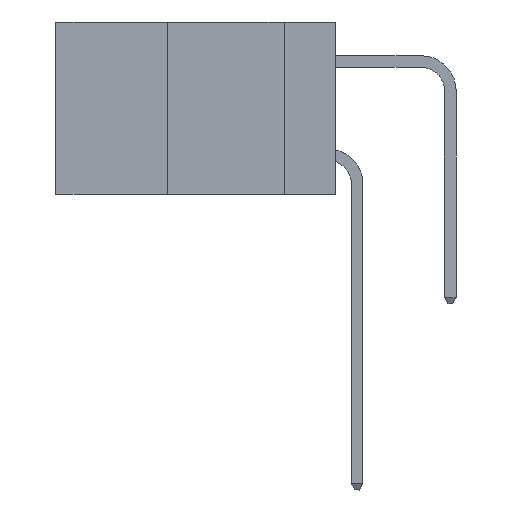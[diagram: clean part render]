
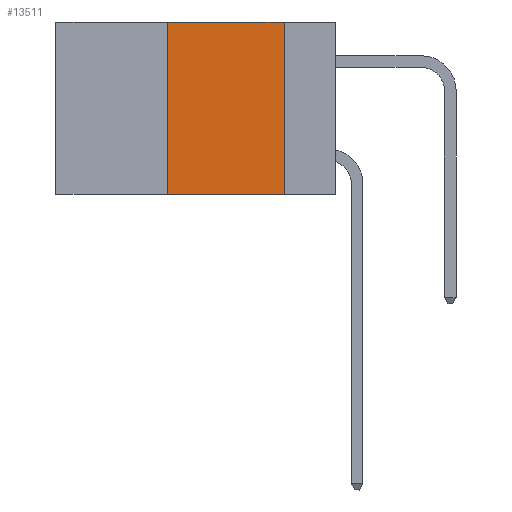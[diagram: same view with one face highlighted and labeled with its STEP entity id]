
A CAD part, left-side view. The second image highlights one B-rep face of the part: STEP entity #13511.
In plain terms, the highlighted planar face has unit normal (-1, 0, 0).
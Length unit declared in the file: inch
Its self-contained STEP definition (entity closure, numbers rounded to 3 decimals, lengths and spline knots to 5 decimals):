
#1411 = EDGE_CURVE ( 'NONE', #8501, #7712, #13005, .T. ) ;
#2580 = CARTESIAN_POINT ( 'NONE',  ( 0., 0.11, 0. ) ) ;
#2696 = LINE ( 'NONE', #4878, #17691 ) ;
#2960 = CARTESIAN_POINT ( 'NONE',  ( 0., 0.6, -0.37 ) ) ;
#3061 = DIRECTION ( 'NONE',  ( 1., 0., 0. ) ) ;
#4762 = AXIS2_PLACEMENT_3D ( 'NONE', #6538, #3061, #13594 ) ;
#4878 = CARTESIAN_POINT ( 'NONE',  ( 0., 0.6, 0. ) ) ;
#6538 = CARTESIAN_POINT ( 'NONE',  ( 0., 0.6, 0. ) ) ;
#7712 = VERTEX_POINT ( 'NONE', #12210 ) ;
#8501 = VERTEX_POINT ( 'NONE', #11268 ) ;
#8573 = DIRECTION ( 'NONE',  ( 0., 0., -1. ) ) ;
#8809 = VERTEX_POINT ( 'NONE', #17375 ) ;
#9532 = EDGE_CURVE ( 'NONE', #8501, #8809, #18796, .T. ) ;
#11268 = CARTESIAN_POINT ( 'NONE',  ( 0., 0.36, -0.37 ) ) ;
#12210 = CARTESIAN_POINT ( 'NONE',  ( 0., 0.36, 0. ) ) ;
#13005 = LINE ( 'NONE', #18202, #14897 ) ;
#13090 = VECTOR ( 'NONE', #8573, 39.37008 ) ;
#13377 = ORIENTED_EDGE ( 'NONE', *, *, #21115, .F. ) ;
#13511 = ADVANCED_FACE ( 'NONE', ( #18684 ), #22386, .F. ) ;
#13594 = DIRECTION ( 'NONE',  ( 0., 0., -1. ) ) ;
#13781 = EDGE_LOOP ( 'NONE', ( #13377, #19821, #18024, #15419 ) ) ;
#13934 = EDGE_CURVE ( 'NONE', #7712, #19516, #2696, .T. ) ;
#14502 = DIRECTION ( 'NONE',  ( 0., 0., 1. ) ) ;
#14897 = VECTOR ( 'NONE', #14502, 39.37008 ) ;
#15069 = DIRECTION ( 'NONE',  ( 0., -1., 0. ) ) ;
#15419 = ORIENTED_EDGE ( 'NONE', *, *, #9532, .T. ) ;
#15630 = CARTESIAN_POINT ( 'NONE',  ( 0., 0.11, 0. ) ) ;
#17073 = DIRECTION ( 'NONE',  ( 0., -1., 0. ) ) ;
#17375 = CARTESIAN_POINT ( 'NONE',  ( 0., 0.11, -0.37 ) ) ;
#17691 = VECTOR ( 'NONE', #15069, 39.37008 ) ;
#18024 = ORIENTED_EDGE ( 'NONE', *, *, #1411, .F. ) ;
#18202 = CARTESIAN_POINT ( 'NONE',  ( 0., 0.36, 0. ) ) ;
#18684 = FACE_OUTER_BOUND ( 'NONE', #13781, .T. ) ;
#18796 = LINE ( 'NONE', #2960, #21257 ) ;
#18987 = LINE ( 'NONE', #15630, #13090 ) ;
#19516 = VERTEX_POINT ( 'NONE', #2580 ) ;
#19821 = ORIENTED_EDGE ( 'NONE', *, *, #13934, .F. ) ;
#21115 = EDGE_CURVE ( 'NONE', #19516, #8809, #18987, .T. ) ;
#21257 = VECTOR ( 'NONE', #17073, 39.37008 ) ;
#22386 = PLANE ( 'NONE',  #4762 ) ;
